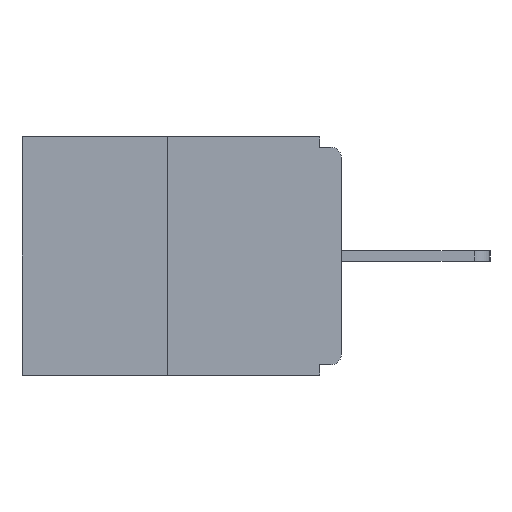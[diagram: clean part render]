
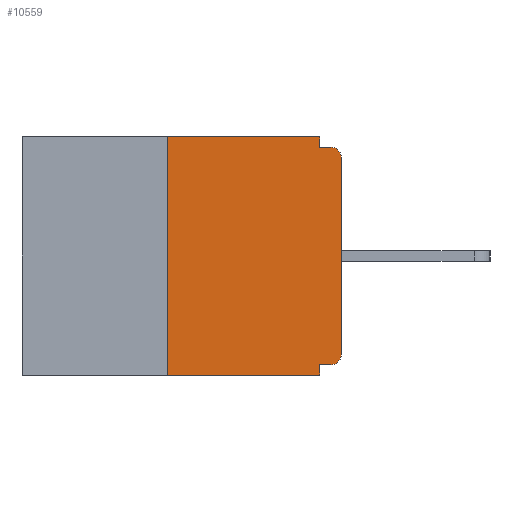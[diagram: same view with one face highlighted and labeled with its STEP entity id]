
A CAD part, left-side view. The second image highlights one B-rep face of the part: STEP entity #10559.
In plain terms, the highlighted planar face has unit normal (-1, 0, 0).
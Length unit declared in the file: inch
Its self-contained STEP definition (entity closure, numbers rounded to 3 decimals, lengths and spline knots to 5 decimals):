
#38 = CARTESIAN_POINT ( 'NONE',  ( 0., 0.031, -0.328 ) ) ;
#56 = CARTESIAN_POINT ( 'NONE',  ( 0., 0.015, -0.015 ) ) ;
#98 = EDGE_CURVE ( 'NONE', #10817, #303, #1678, .T. ) ;
#267 = EDGE_CURVE ( 'NONE', #4766, #4976, #382, .T. ) ;
#303 = VERTEX_POINT ( 'NONE', #10765 ) ;
#340 = CARTESIAN_POINT ( 'NONE',  ( 0., 0.015, -0.03 ) ) ;
#382 = LINE ( 'NONE', #11359, #2469 ) ;
#631 = ORIENTED_EDGE ( 'NONE', *, *, #3994, .T. ) ;
#886 = VECTOR ( 'NONE', #9930, 39.37008 ) ;
#1308 = DIRECTION ( 'NONE',  ( 0., -1., 0. ) ) ;
#1329 = LINE ( 'NONE', #8418, #9077 ) ;
#1373 = DIRECTION ( 'NONE',  ( 0., 0., -1. ) ) ;
#1396 = CARTESIAN_POINT ( 'NONE',  ( 0., 0.015, -0.313 ) ) ;
#1498 = DIRECTION ( 'NONE',  ( 1., 0., 0. ) ) ;
#1636 = EDGE_CURVE ( 'NONE', #6578, #7269, #1329, .T. ) ;
#1661 = CARTESIAN_POINT ( 'NONE',  ( 0., 0.031, -0.343 ) ) ;
#1678 = LINE ( 'NONE', #7667, #12031 ) ;
#1766 = LINE ( 'NONE', #9101, #4401 ) ;
#1776 = EDGE_LOOP ( 'NONE', ( #12099, #2070, #12702, #2384, #2704, #5351, #3012, #631, #8705, #11333 ) ) ;
#2070 = ORIENTED_EDGE ( 'NONE', *, *, #4302, .F. ) ;
#2114 = FACE_OUTER_BOUND ( 'NONE', #1776, .T. ) ;
#2384 = ORIENTED_EDGE ( 'NONE', *, *, #11973, .F. ) ;
#2429 = DIRECTION ( 'NONE',  ( 0., 0., -1. ) ) ;
#2469 = VECTOR ( 'NONE', #4787, 39.37008 ) ;
#2537 = DIRECTION ( 'NONE',  ( 0., -1., 0. ) ) ;
#2618 = AXIS2_PLACEMENT_3D ( 'NONE', #11499, #1498, #8572 ) ;
#2704 = ORIENTED_EDGE ( 'NONE', *, *, #267, .F. ) ;
#2855 = VECTOR ( 'NONE', #1308, 39.37008 ) ;
#2924 = CARTESIAN_POINT ( 'NONE',  ( 0., 0.031, 0. ) ) ;
#3012 = ORIENTED_EDGE ( 'NONE', *, *, #98, .T. ) ;
#3055 = DIRECTION ( 'NONE',  ( 0., 0., -1. ) ) ;
#3473 = PLANE ( 'NONE',  #2618 ) ;
#3916 = CARTESIAN_POINT ( 'NONE',  ( 0., 0.25, 0. ) ) ;
#3994 = EDGE_CURVE ( 'NONE', #303, #6302, #12650, .T. ) ;
#4009 = VERTEX_POINT ( 'NONE', #12361 ) ;
#4302 = EDGE_CURVE ( 'NONE', #6578, #5947, #11266, .T. ) ;
#4401 = VECTOR ( 'NONE', #3055, 39.37008 ) ;
#4766 = VERTEX_POINT ( 'NONE', #12778 ) ;
#4787 = DIRECTION ( 'NONE',  ( 0., 1., 0. ) ) ;
#4855 = CARTESIAN_POINT ( 'NONE',  ( 0., 0., -0.313 ) ) ;
#4976 = VERTEX_POINT ( 'NONE', #38 ) ;
#5262 = EDGE_CURVE ( 'NONE', #4766, #10817, #10604, .T. ) ;
#5351 = ORIENTED_EDGE ( 'NONE', *, *, #5262, .T. ) ;
#5505 = VECTOR ( 'NONE', #9934, 39.37008 ) ;
#5507 = LINE ( 'NONE', #12301, #2855 ) ;
#5947 = VERTEX_POINT ( 'NONE', #9558 ) ;
#6302 = VERTEX_POINT ( 'NONE', #56 ) ;
#6578 = VERTEX_POINT ( 'NONE', #9543 ) ;
#6638 = DIRECTION ( 'NONE',  ( 0., -1., 0. ) ) ;
#7269 = VERTEX_POINT ( 'NONE', #1661 ) ;
#7420 = DIRECTION ( 'NONE',  ( -1., 0., 0. ) ) ;
#7591 = LINE ( 'NONE', #2924, #5505 ) ;
#7622 = CARTESIAN_POINT ( 'NONE',  ( 0., 0.46, 0. ) ) ;
#7667 = CARTESIAN_POINT ( 'NONE',  ( 0., 0., 0. ) ) ;
#7735 = EDGE_CURVE ( 'NONE', #5947, #8982, #10370, .T. ) ;
#7986 = EDGE_CURVE ( 'NONE', #8982, #4009, #7591, .T. ) ;
#8159 = AXIS2_PLACEMENT_3D ( 'NONE', #1396, #8481, #2429 ) ;
#8418 = CARTESIAN_POINT ( 'NONE',  ( 0., 0.46, -0.343 ) ) ;
#8481 = DIRECTION ( 'NONE',  ( -1., 0., 0. ) ) ;
#8572 = DIRECTION ( 'NONE',  ( 0., 0., -1. ) ) ;
#8675 = EDGE_CURVE ( 'NONE', #4009, #6302, #5507, .T. ) ;
#8704 = VECTOR ( 'NONE', #2537, 39.37008 ) ;
#8705 = ORIENTED_EDGE ( 'NONE', *, *, #8675, .F. ) ;
#8982 = VERTEX_POINT ( 'NONE', #11786 ) ;
#9077 = VECTOR ( 'NONE', #6638, 39.37008 ) ;
#9101 = CARTESIAN_POINT ( 'NONE',  ( 0., 0.031, -0.343 ) ) ;
#9543 = CARTESIAN_POINT ( 'NONE',  ( 0., 0.25, -0.343 ) ) ;
#9558 = CARTESIAN_POINT ( 'NONE',  ( 0., 0.25, 0. ) ) ;
#9930 = DIRECTION ( 'NONE',  ( 0., 0., 1. ) ) ;
#9934 = DIRECTION ( 'NONE',  ( 0., 0., -1. ) ) ;
#10370 = LINE ( 'NONE', #7622, #8704 ) ;
#10559 = ADVANCED_FACE ( 'NONE', ( #2114 ), #3473, .F. ) ;
#10604 = CIRCLE ( 'NONE', #8159, 0.015 ) ;
#10765 = CARTESIAN_POINT ( 'NONE',  ( 0., 0., -0.03 ) ) ;
#10817 = VERTEX_POINT ( 'NONE', #4855 ) ;
#11266 = LINE ( 'NONE', #3916, #886 ) ;
#11333 = ORIENTED_EDGE ( 'NONE', *, *, #7986, .F. ) ;
#11359 = CARTESIAN_POINT ( 'NONE',  ( 0., 0., -0.328 ) ) ;
#11499 = CARTESIAN_POINT ( 'NONE',  ( 0., 0.46, 0. ) ) ;
#11786 = CARTESIAN_POINT ( 'NONE',  ( 0., 0.031, 0. ) ) ;
#11973 = EDGE_CURVE ( 'NONE', #4976, #7269, #1766, .T. ) ;
#12031 = VECTOR ( 'NONE', #12937, 39.37008 ) ;
#12099 = ORIENTED_EDGE ( 'NONE', *, *, #7735, .F. ) ;
#12301 = CARTESIAN_POINT ( 'NONE',  ( 0., 0., -0.015 ) ) ;
#12361 = CARTESIAN_POINT ( 'NONE',  ( 0., 0.031, -0.015 ) ) ;
#12650 = CIRCLE ( 'NONE', #12677, 0.015 ) ;
#12677 = AXIS2_PLACEMENT_3D ( 'NONE', #340, #7420, #1373 ) ;
#12702 = ORIENTED_EDGE ( 'NONE', *, *, #1636, .T. ) ;
#12778 = CARTESIAN_POINT ( 'NONE',  ( 0., 0.015, -0.328 ) ) ;
#12937 = DIRECTION ( 'NONE',  ( 0., 0., 1. ) ) ;
